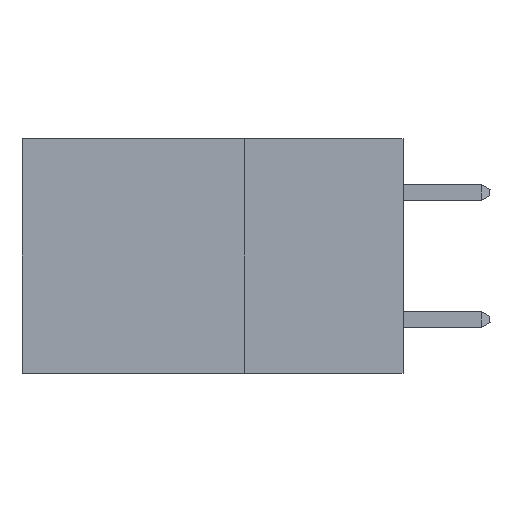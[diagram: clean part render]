
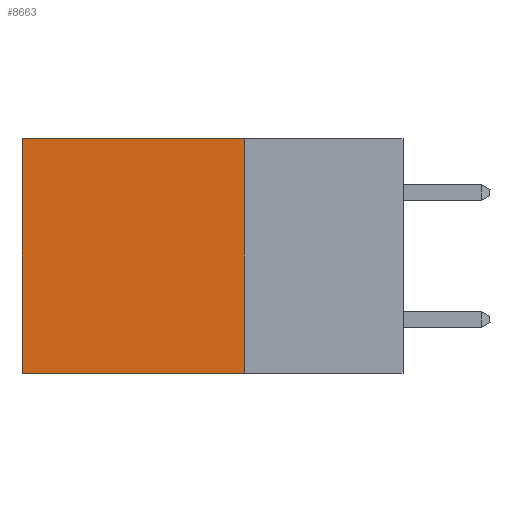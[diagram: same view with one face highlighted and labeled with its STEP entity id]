
A CAD part, left-side view. The second image highlights one B-rep face of the part: STEP entity #8663.
In plain terms, the highlighted planar face has unit normal (-1, 0, 0).
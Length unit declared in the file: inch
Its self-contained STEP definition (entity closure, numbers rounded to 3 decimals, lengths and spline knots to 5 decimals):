
#163 = ORIENTED_EDGE ( 'NONE', *, *, #26049, .F. ) ;
#622 = DIRECTION ( 'NONE',  ( 0., 0., -1. ) ) ;
#1535 = VECTOR ( 'NONE', #22622, 39.37008 ) ;
#2186 = CARTESIAN_POINT ( 'NONE',  ( 0.2875, 0.6, 0. ) ) ;
#3056 = EDGE_CURVE ( 'NONE', #35907, #28189, #20892, .T. ) ;
#3936 = CARTESIAN_POINT ( 'NONE',  ( 0.2875, 0.25, 0. ) ) ;
#4416 = VECTOR ( 'NONE', #18316, 39.37008 ) ;
#4462 = LINE ( 'NONE', #16112, #8399 ) ;
#7775 = VERTEX_POINT ( 'NONE', #2186 ) ;
#8037 = CARTESIAN_POINT ( 'NONE',  ( 0.2875, 0.25, -0.37 ) ) ;
#8316 = VERTEX_POINT ( 'NONE', #18411 ) ;
#8399 = VECTOR ( 'NONE', #622, 39.37008 ) ;
#8540 = FACE_OUTER_BOUND ( 'NONE', #27746, .T. ) ;
#8663 = ADVANCED_FACE ( 'NONE', ( #8540 ), #38425, .F. ) ;
#13818 = DIRECTION ( 'NONE',  ( 1., 0., 0. ) ) ;
#14525 = AXIS2_PLACEMENT_3D ( 'NONE', #40044, #13818, #33794 ) ;
#16112 = CARTESIAN_POINT ( 'NONE',  ( 0.2875, 0.6, 0. ) ) ;
#16363 = VECTOR ( 'NONE', #32948, 39.37008 ) ;
#18316 = DIRECTION ( 'NONE',  ( 0., 1., 0. ) ) ;
#18411 = CARTESIAN_POINT ( 'NONE',  ( 0.2875, 0.25, 0. ) ) ;
#19523 = CARTESIAN_POINT ( 'NONE',  ( 0.2875, 0.6, -0.37 ) ) ;
#20892 = LINE ( 'NONE', #8037, #4416 ) ;
#22622 = DIRECTION ( 'NONE',  ( 0., 1., 0. ) ) ;
#24079 = EDGE_CURVE ( 'NONE', #8316, #7775, #29233, .T. ) ;
#26049 = EDGE_CURVE ( 'NONE', #8316, #35907, #32979, .T. ) ;
#27746 = EDGE_LOOP ( 'NONE', ( #32966, #33326, #163, #29721 ) ) ;
#28189 = VERTEX_POINT ( 'NONE', #19523 ) ;
#29233 = LINE ( 'NONE', #3936, #1535 ) ;
#29721 = ORIENTED_EDGE ( 'NONE', *, *, #24079, .T. ) ;
#29942 = CARTESIAN_POINT ( 'NONE',  ( 0.2875, 0.25, 0. ) ) ;
#30483 = EDGE_CURVE ( 'NONE', #7775, #28189, #4462, .T. ) ;
#32948 = DIRECTION ( 'NONE',  ( 0., 0., -1. ) ) ;
#32966 = ORIENTED_EDGE ( 'NONE', *, *, #30483, .T. ) ;
#32979 = LINE ( 'NONE', #29942, #16363 ) ;
#33326 = ORIENTED_EDGE ( 'NONE', *, *, #3056, .F. ) ;
#33794 = DIRECTION ( 'NONE',  ( 0., 0., -1. ) ) ;
#35907 = VERTEX_POINT ( 'NONE', #39510 ) ;
#38425 = PLANE ( 'NONE',  #14525 ) ;
#39510 = CARTESIAN_POINT ( 'NONE',  ( 0.2875, 0.25, -0.37 ) ) ;
#40044 = CARTESIAN_POINT ( 'NONE',  ( 0.2875, 0.25, 0. ) ) ;
